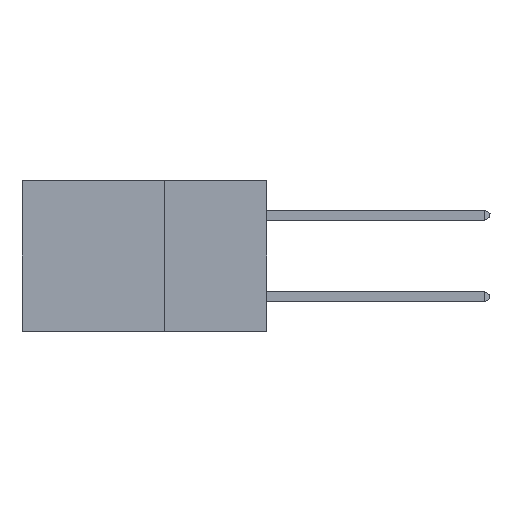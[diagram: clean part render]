
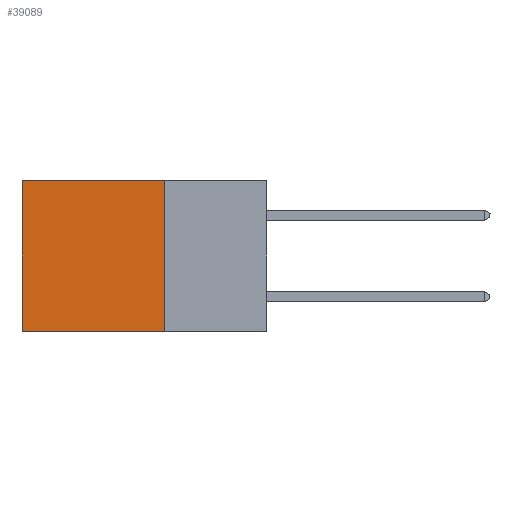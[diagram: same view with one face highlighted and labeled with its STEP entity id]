
A CAD part, left-side view. The second image highlights one B-rep face of the part: STEP entity #39089.
In plain terms, the highlighted planar face has unit normal (-1, 0, 0).
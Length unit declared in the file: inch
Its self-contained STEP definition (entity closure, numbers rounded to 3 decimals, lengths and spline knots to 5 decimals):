
#1391 = VERTEX_POINT ( 'NONE', #38418 ) ;
#2225 = LINE ( 'NONE', #21922, #10290 ) ;
#2717 = LINE ( 'NONE', #33209, #10794 ) ;
#4830 = DIRECTION ( 'NONE',  ( 0., 1., 0. ) ) ;
#7085 = CARTESIAN_POINT ( 'NONE',  ( 0.2875, 0.6, 0. ) ) ;
#9320 = VECTOR ( 'NONE', #34165, 39.37008 ) ;
#9413 = DIRECTION ( 'NONE',  ( 0., 1., 0. ) ) ;
#10290 = VECTOR ( 'NONE', #4830, 39.37008 ) ;
#10481 = ORIENTED_EDGE ( 'NONE', *, *, #15773, .T. ) ;
#10794 = VECTOR ( 'NONE', #9413, 39.37008 ) ;
#10953 = EDGE_CURVE ( 'NONE', #28371, #16650, #17375, .T. ) ;
#11096 = EDGE_LOOP ( 'NONE', ( #42014, #41147, #37198, #10481 ) ) ;
#15773 = EDGE_CURVE ( 'NONE', #1391, #28371, #2717, .T. ) ;
#16650 = VERTEX_POINT ( 'NONE', #27569 ) ;
#17375 = LINE ( 'NONE', #7085, #9320 ) ;
#21019 = DIRECTION ( 'NONE',  ( 0., 0., -1. ) ) ;
#21108 = AXIS2_PLACEMENT_3D ( 'NONE', #37807, #41140, #21019 ) ;
#21922 = CARTESIAN_POINT ( 'NONE',  ( 0.2875, 0.25, -0.37 ) ) ;
#22876 = VERTEX_POINT ( 'NONE', #32951 ) ;
#23643 = DIRECTION ( 'NONE',  ( 0., 0., -1. ) ) ;
#25504 = CARTESIAN_POINT ( 'NONE',  ( 0.2875, 0.6, 0. ) ) ;
#27236 = VECTOR ( 'NONE', #23643, 39.37008 ) ;
#27569 = CARTESIAN_POINT ( 'NONE',  ( 0.2875, 0.6, -0.37 ) ) ;
#28324 = EDGE_CURVE ( 'NONE', #22876, #16650, #2225, .T. ) ;
#28371 = VERTEX_POINT ( 'NONE', #25504 ) ;
#30433 = CARTESIAN_POINT ( 'NONE',  ( 0.2875, 0.25, 0. ) ) ;
#30828 = EDGE_CURVE ( 'NONE', #1391, #22876, #36148, .T. ) ;
#31060 = PLANE ( 'NONE',  #21108 ) ;
#32951 = CARTESIAN_POINT ( 'NONE',  ( 0.2875, 0.25, -0.37 ) ) ;
#33209 = CARTESIAN_POINT ( 'NONE',  ( 0.2875, 0.25, 0. ) ) ;
#33496 = FACE_OUTER_BOUND ( 'NONE', #11096, .T. ) ;
#34165 = DIRECTION ( 'NONE',  ( 0., 0., -1. ) ) ;
#36148 = LINE ( 'NONE', #30433, #27236 ) ;
#37198 = ORIENTED_EDGE ( 'NONE', *, *, #30828, .F. ) ;
#37807 = CARTESIAN_POINT ( 'NONE',  ( 0.2875, 0.25, 0. ) ) ;
#38418 = CARTESIAN_POINT ( 'NONE',  ( 0.2875, 0.25, 0. ) ) ;
#39089 = ADVANCED_FACE ( 'NONE', ( #33496 ), #31060, .F. ) ;
#41140 = DIRECTION ( 'NONE',  ( 1., 0., 0. ) ) ;
#41147 = ORIENTED_EDGE ( 'NONE', *, *, #28324, .F. ) ;
#42014 = ORIENTED_EDGE ( 'NONE', *, *, #10953, .T. ) ;
